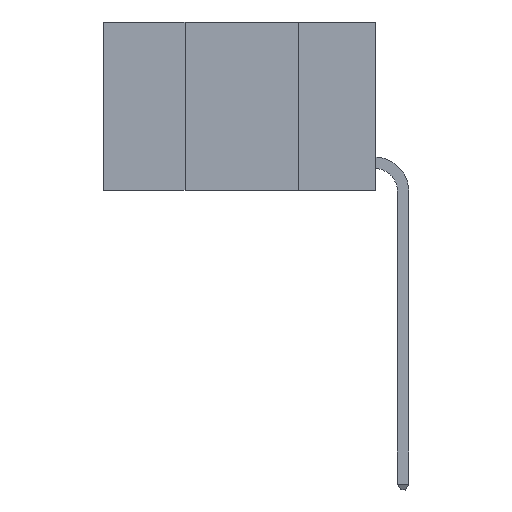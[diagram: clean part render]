
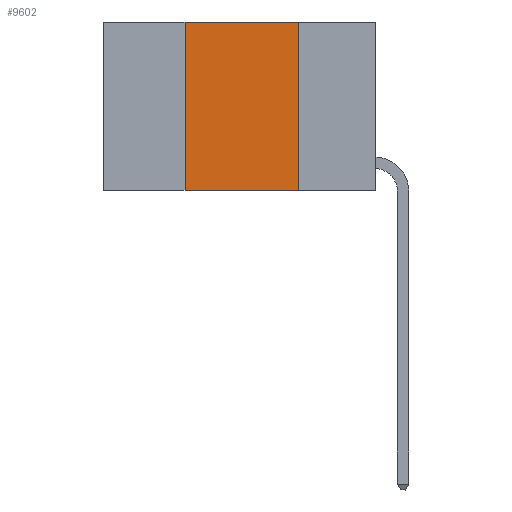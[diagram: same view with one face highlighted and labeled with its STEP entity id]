
A CAD part, left-side view. The second image highlights one B-rep face of the part: STEP entity #9602.
In plain terms, the highlighted planar face has unit normal (-1, 0, 0).
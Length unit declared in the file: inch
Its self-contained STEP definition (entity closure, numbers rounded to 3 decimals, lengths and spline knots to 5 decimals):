
#279 = LINE ( 'NONE', #11306, #5103 ) ;
#457 = DIRECTION ( 'NONE',  ( 0., 0., -1. ) ) ;
#1155 = VERTEX_POINT ( 'NONE', #6159 ) ;
#1505 = CARTESIAN_POINT ( 'NONE',  ( 0., 0.6, 0. ) ) ;
#1884 = EDGE_CURVE ( 'NONE', #5274, #3237, #10502, .T. ) ;
#1901 = EDGE_CURVE ( 'NONE', #11182, #1155, #279, .T. ) ;
#2110 = LINE ( 'NONE', #8961, #11952 ) ;
#2206 = EDGE_CURVE ( 'NONE', #5274, #11182, #2110, .T. ) ;
#2470 = PLANE ( 'NONE',  #5506 ) ;
#2855 = VECTOR ( 'NONE', #6058, 39.37008 ) ;
#2872 = LINE ( 'NONE', #6264, #4123 ) ;
#3081 = CARTESIAN_POINT ( 'NONE',  ( 0., 0.17, -0.37 ) ) ;
#3237 = VERTEX_POINT ( 'NONE', #3081 ) ;
#4123 = VECTOR ( 'NONE', #457, 39.37008 ) ;
#4424 = DIRECTION ( 'NONE',  ( 0., 0., -1. ) ) ;
#4884 = FACE_OUTER_BOUND ( 'NONE', #10671, .T. ) ;
#5103 = VECTOR ( 'NONE', #8281, 39.37008 ) ;
#5274 = VERTEX_POINT ( 'NONE', #9988 ) ;
#5506 = AXIS2_PLACEMENT_3D ( 'NONE', #1505, #10150, #4424 ) ;
#5914 = ORIENTED_EDGE ( 'NONE', *, *, #2206, .F. ) ;
#6058 = DIRECTION ( 'NONE',  ( 0., -1., 0. ) ) ;
#6159 = CARTESIAN_POINT ( 'NONE',  ( 0., 0.17, 0. ) ) ;
#6264 = CARTESIAN_POINT ( 'NONE',  ( 0., 0.17, 0. ) ) ;
#7717 = ORIENTED_EDGE ( 'NONE', *, *, #1901, .F. ) ;
#8281 = DIRECTION ( 'NONE',  ( 0., -1., 0. ) ) ;
#8648 = DIRECTION ( 'NONE',  ( 0., 0., 1. ) ) ;
#8961 = CARTESIAN_POINT ( 'NONE',  ( 0., 0.42, 0. ) ) ;
#9602 = ADVANCED_FACE ( 'NONE', ( #4884 ), #2470, .F. ) ;
#9988 = CARTESIAN_POINT ( 'NONE',  ( 0., 0.42, -0.37 ) ) ;
#10019 = CARTESIAN_POINT ( 'NONE',  ( 0., 0.6, -0.37 ) ) ;
#10150 = DIRECTION ( 'NONE',  ( 1., 0., 0. ) ) ;
#10502 = LINE ( 'NONE', #10019, #2855 ) ;
#10671 = EDGE_LOOP ( 'NONE', ( #11843, #7717, #5914, #12006 ) ) ;
#10790 = CARTESIAN_POINT ( 'NONE',  ( 0., 0.42, 0. ) ) ;
#11182 = VERTEX_POINT ( 'NONE', #10790 ) ;
#11306 = CARTESIAN_POINT ( 'NONE',  ( 0., 0.6, 0. ) ) ;
#11312 = EDGE_CURVE ( 'NONE', #1155, #3237, #2872, .T. ) ;
#11843 = ORIENTED_EDGE ( 'NONE', *, *, #11312, .F. ) ;
#11952 = VECTOR ( 'NONE', #8648, 39.37008 ) ;
#12006 = ORIENTED_EDGE ( 'NONE', *, *, #1884, .T. ) ;
